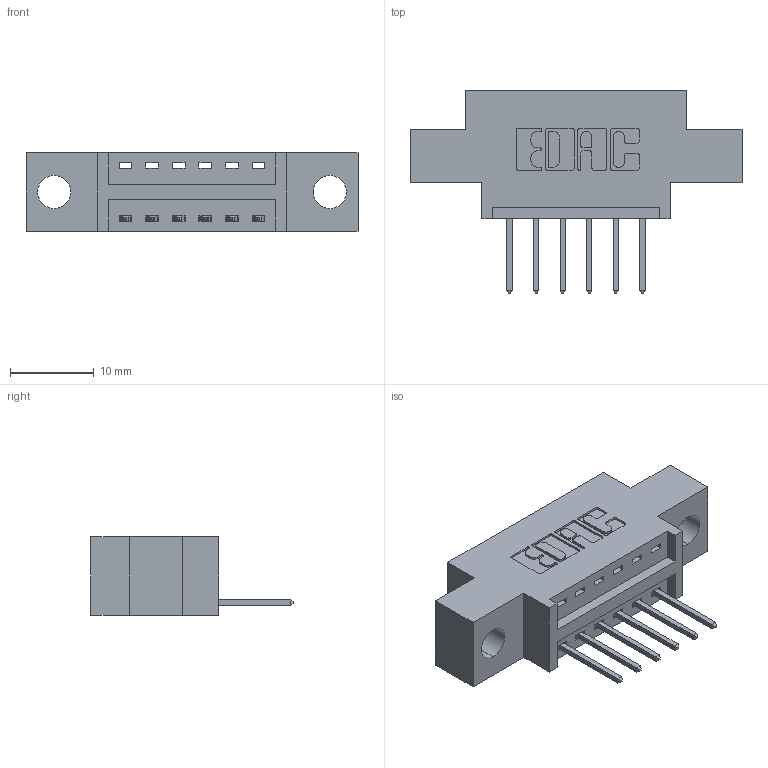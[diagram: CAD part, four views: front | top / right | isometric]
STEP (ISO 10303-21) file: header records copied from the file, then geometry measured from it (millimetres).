
FILE_DESCRIPTION (( 'STEP AP203' ), '1' );
FILE_NAME ('396-006-526-604.STEP', '2022-05-17T06:15:46', ( '' ), ( '' ), 'SwSTEP 2.0', 'SolidWorks 2020', '' );
FILE_SCHEMA (( 'CONFIG_CONTROL_DESIGN' ));
Length unit declared in the file: inch
Products named in the file (3): 345-292-001_345-293-126; 396-006-526-604; 346 Part_0.170 Offset - 0.156 Dia-TH
Assembly tree (7 placements, depth 2):
  396-006-526-604
    346 Part_0.170 Offset - 0.156 Dia-TH
    345-292-001_345-293-126  x6
Bounding box: 39.62 x 24.13 x 9.4 mm (x, y, z)
Volume: 3279.5 mm3; surface area: 3702.3 mm2
Topology: 7 solids, 7 shells, 488 faces, 1433 edges, 946 vertices
Faces by surface type: plane 334, cylinder 154
Entity records: 9139 total; most frequent: CARTESIAN_POINT 1588, ORIENTED_EDGE 1526, DIRECTION 1443, EDGE_CURVE 763, LINE 607, VECTOR 607, VERTEX_POINT 506, AXIS2_PLACEMENT_3D 418
